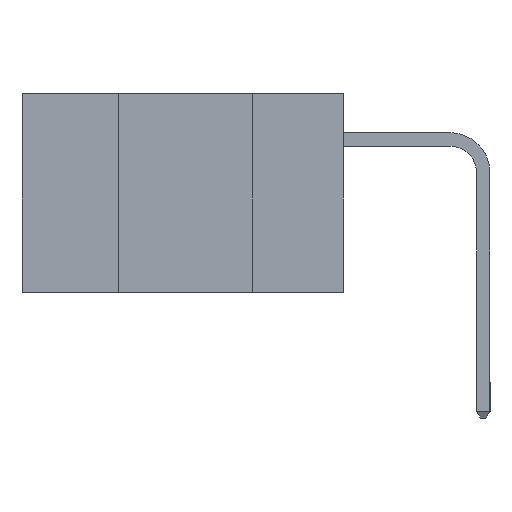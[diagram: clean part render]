
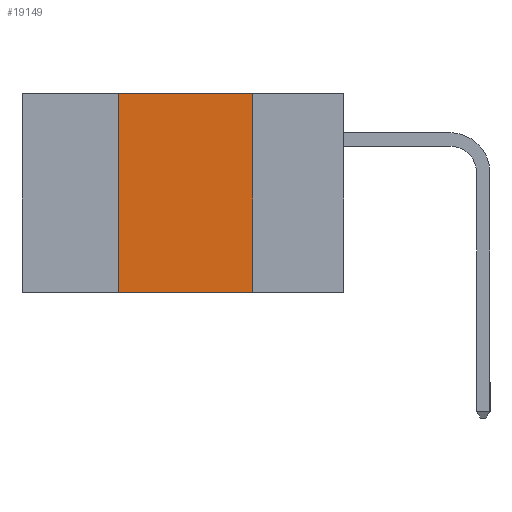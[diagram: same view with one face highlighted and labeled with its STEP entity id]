
A CAD part, left-side view. The second image highlights one B-rep face of the part: STEP entity #19149.
In plain terms, the highlighted planar face has unit normal (-1, 0, 0).
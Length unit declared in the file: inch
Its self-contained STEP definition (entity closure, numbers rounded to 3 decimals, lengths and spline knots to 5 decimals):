
#374 = VERTEX_POINT ( 'NONE', #9152 ) ;
#485 = EDGE_CURVE ( 'NONE', #5956, #19491, #15991, .T. ) ;
#597 = EDGE_CURVE ( 'NONE', #19491, #374, #22879, .T. ) ;
#809 = DIRECTION ( 'NONE',  ( 1., 0., 0. ) ) ;
#836 = VECTOR ( 'NONE', #9015, 39.37008 ) ;
#2311 = ORIENTED_EDGE ( 'NONE', *, *, #485, .F. ) ;
#2733 = EDGE_CURVE ( 'NONE', #16085, #5956, #16288, .T. ) ;
#3581 = CARTESIAN_POINT ( 'NONE',  ( 0., 0.42, 0. ) ) ;
#4764 = FACE_OUTER_BOUND ( 'NONE', #19390, .T. ) ;
#4815 = DIRECTION ( 'NONE',  ( 0., -1., 0. ) ) ;
#4878 = PLANE ( 'NONE',  #22088 ) ;
#5956 = VERTEX_POINT ( 'NONE', #3581 ) ;
#6570 = LINE ( 'NONE', #13667, #9737 ) ;
#8780 = CARTESIAN_POINT ( 'NONE',  ( 0., 0.17, -0.37 ) ) ;
#9015 = DIRECTION ( 'NONE',  ( 0., -1., 0. ) ) ;
#9152 = CARTESIAN_POINT ( 'NONE',  ( 0., 0.17, -0.37 ) ) ;
#9737 = VECTOR ( 'NONE', #4815, 39.37008 ) ;
#9866 = CARTESIAN_POINT ( 'NONE',  ( 0., 0.17, 0. ) ) ;
#11179 = CARTESIAN_POINT ( 'NONE',  ( 0., 0.42, -0.37 ) ) ;
#11425 = ORIENTED_EDGE ( 'NONE', *, *, #597, .F. ) ;
#12258 = ORIENTED_EDGE ( 'NONE', *, *, #2733, .F. ) ;
#12533 = CARTESIAN_POINT ( 'NONE',  ( 0., 0.6, 0. ) ) ;
#13667 = CARTESIAN_POINT ( 'NONE',  ( 0., 0.6, -0.37 ) ) ;
#15702 = VECTOR ( 'NONE', #21035, 39.37008 ) ;
#15991 = LINE ( 'NONE', #12533, #836 ) ;
#16085 = VERTEX_POINT ( 'NONE', #22184 ) ;
#16288 = LINE ( 'NONE', #11179, #21742 ) ;
#16644 = ORIENTED_EDGE ( 'NONE', *, *, #17095, .T. ) ;
#16742 = DIRECTION ( 'NONE',  ( 0., 0., -1. ) ) ;
#17095 = EDGE_CURVE ( 'NONE', #16085, #374, #6570, .T. ) ;
#19149 = ADVANCED_FACE ( 'NONE', ( #4764 ), #4878, .F. ) ;
#19390 = EDGE_LOOP ( 'NONE', ( #11425, #2311, #12258, #16644 ) ) ;
#19491 = VERTEX_POINT ( 'NONE', #9866 ) ;
#21035 = DIRECTION ( 'NONE',  ( 0., 0., -1. ) ) ;
#21742 = VECTOR ( 'NONE', #21804, 39.37008 ) ;
#21804 = DIRECTION ( 'NONE',  ( 0., 0., 1. ) ) ;
#22088 = AXIS2_PLACEMENT_3D ( 'NONE', #22602, #809, #16742 ) ;
#22184 = CARTESIAN_POINT ( 'NONE',  ( 0., 0.42, -0.37 ) ) ;
#22602 = CARTESIAN_POINT ( 'NONE',  ( 0., 0.6, 0. ) ) ;
#22879 = LINE ( 'NONE', #8780, #15702 ) ;
